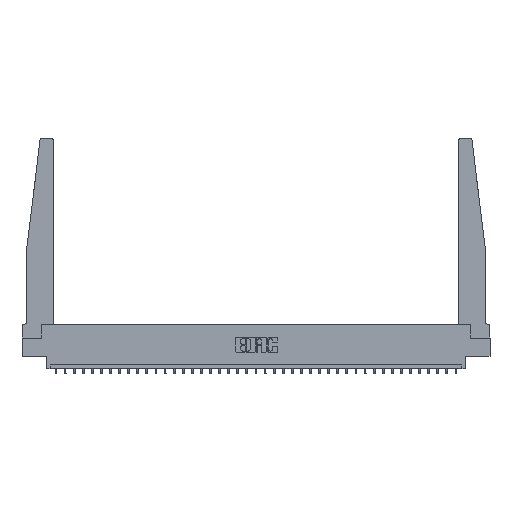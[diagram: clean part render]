
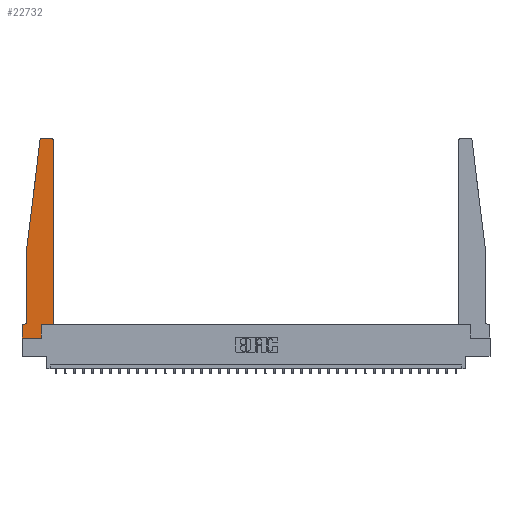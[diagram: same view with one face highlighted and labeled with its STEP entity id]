
A CAD part, top view. The second image highlights one B-rep face of the part: STEP entity #22732.
In plain terms, the highlighted planar face has unit normal (0, 0, 1).
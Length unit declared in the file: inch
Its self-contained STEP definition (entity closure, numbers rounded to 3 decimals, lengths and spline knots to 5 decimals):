
#121 = CARTESIAN_POINT ( 'NONE',  ( 0.425, 0.18, 0.37 ) ) ;
#273 = LINE ( 'NONE', #121, #26267 ) ;
#359 = ORIENTED_EDGE ( 'NONE', *, *, #1208, .T. ) ;
#466 = VERTEX_POINT ( 'NONE', #6820 ) ;
#1101 = LINE ( 'NONE', #6341, #20397 ) ;
#1208 = EDGE_CURVE ( 'NONE', #28854, #10786, #15111, .T. ) ;
#1490 = VERTEX_POINT ( 'NONE', #4313 ) ;
#1875 = CARTESIAN_POINT ( 'NONE',  ( 0.065, 0.2375, 0.37 ) ) ;
#2085 = CARTESIAN_POINT ( 'NONE',  ( 0., 0., 0.37 ) ) ;
#2220 = DIRECTION ( 'NONE',  ( 0., 1., 0. ) ) ;
#2497 = VERTEX_POINT ( 'NONE', #21222 ) ;
#3133 = CARTESIAN_POINT ( 'NONE',  ( 0., 0., 0.37 ) ) ;
#3214 = CARTESIAN_POINT ( 'NONE',  ( 0., 0., 0.37 ) ) ;
#3490 = ORIENTED_EDGE ( 'NONE', *, *, #5135, .T. ) ;
#3610 = VERTEX_POINT ( 'NONE', #25911 ) ;
#3616 = LINE ( 'NONE', #13881, #29569 ) ;
#3921 = DIRECTION ( 'NONE',  ( -1., 0., 0. ) ) ;
#4313 = CARTESIAN_POINT ( 'NONE',  ( 0.425, 0.18, 0.37 ) ) ;
#4777 = EDGE_CURVE ( 'NONE', #13607, #4840, #18002, .T. ) ;
#4840 = VERTEX_POINT ( 'NONE', #18694 ) ;
#4841 = ORIENTED_EDGE ( 'NONE', *, *, #30236, .T. ) ;
#5081 = CARTESIAN_POINT ( 'NONE',  ( 0.425, 2.72, 0.37 ) ) ;
#5135 = EDGE_CURVE ( 'NONE', #13281, #1490, #273, .T. ) ;
#5144 = ORIENTED_EDGE ( 'NONE', *, *, #21351, .T. ) ;
#5397 = CARTESIAN_POINT ( 'NONE',  ( 0.25, 2.75, 0.37 ) ) ;
#5709 = FACE_OUTER_BOUND ( 'NONE', #6802, .T. ) ;
#5917 = AXIS2_PLACEMENT_3D ( 'NONE', #26111, #11046, #28576 ) ;
#6341 = CARTESIAN_POINT ( 'NONE',  ( 0.065, 0.1875, 0.37 ) ) ;
#6802 = EDGE_LOOP ( 'NONE', ( #18828, #26869, #4841, #10801, #17477, #5144, #359, #13051, #18697, #3490, #19641, #19164 ) ) ;
#6820 = CARTESIAN_POINT ( 'NONE',  ( 0.2605, 0., 0.37 ) ) ;
#7043 = EDGE_CURVE ( 'NONE', #19220, #19482, #12801, .T. ) ;
#7483 = EDGE_CURVE ( 'NONE', #466, #13281, #32360, .T. ) ;
#7883 = VECTOR ( 'NONE', #22248, 39.37008 ) ;
#8408 = VECTOR ( 'NONE', #30812, 39.37008 ) ;
#8922 = DIRECTION ( 'NONE',  ( -0.122, -0.992, 0. ) ) ;
#9747 = CARTESIAN_POINT ( 'NONE',  ( 0.2605, 0.18, 0.37 ) ) ;
#10602 = AXIS2_PLACEMENT_3D ( 'NONE', #28550, #13560, #31067 ) ;
#10786 = VERTEX_POINT ( 'NONE', #3214 ) ;
#10801 = ORIENTED_EDGE ( 'NONE', *, *, #12232, .T. ) ;
#11046 = DIRECTION ( 'NONE',  ( 0., 0., -1. ) ) ;
#11524 = CARTESIAN_POINT ( 'NONE',  ( 0.425, 0.18, 0.37 ) ) ;
#12232 = EDGE_CURVE ( 'NONE', #3610, #13607, #22268, .T. ) ;
#12317 = VECTOR ( 'NONE', #21481, 39.37008 ) ;
#12801 = CIRCLE ( 'NONE', #15674, 0.03 ) ;
#12900 = DIRECTION ( 'NONE',  ( 0., 0., 1. ) ) ;
#13051 = ORIENTED_EDGE ( 'NONE', *, *, #31712, .T. ) ;
#13281 = VERTEX_POINT ( 'NONE', #30691 ) ;
#13484 = CARTESIAN_POINT ( 'NONE',  ( 0., 0.1875, 0.37 ) ) ;
#13560 = DIRECTION ( 'NONE',  ( 0., 0., 1. ) ) ;
#13607 = VERTEX_POINT ( 'NONE', #1875 ) ;
#13873 = EDGE_CURVE ( 'NONE', #2497, #19220, #22214, .T. ) ;
#13881 = CARTESIAN_POINT ( 'NONE',  ( 0.065, 1.25, 0.37 ) ) ;
#13954 = VECTOR ( 'NONE', #30551, 39.37008 ) ;
#13956 = CARTESIAN_POINT ( 'NONE',  ( 0.065, 1.25, 0.37 ) ) ;
#14782 = CARTESIAN_POINT ( 'NONE',  ( 0., 0.1875, 0.37 ) ) ;
#15111 = LINE ( 'NONE', #3133, #8408 ) ;
#15674 = AXIS2_PLACEMENT_3D ( 'NONE', #27889, #12900, #30377 ) ;
#16913 = LINE ( 'NONE', #2085, #7883 ) ;
#17211 = CARTESIAN_POINT ( 'NONE',  ( 0.27653, 2.75, 0.37 ) ) ;
#17277 = DIRECTION ( 'NONE',  ( 1., 0., 0. ) ) ;
#17477 = ORIENTED_EDGE ( 'NONE', *, *, #4777, .T. ) ;
#18002 = CIRCLE ( 'NONE', #5917, 0.05 ) ;
#18322 = EDGE_CURVE ( 'NONE', #25398, #2497, #27342, .T. ) ;
#18694 = CARTESIAN_POINT ( 'NONE',  ( 0.015, 0.1875, 0.37 ) ) ;
#18697 = ORIENTED_EDGE ( 'NONE', *, *, #7483, .T. ) ;
#18828 = ORIENTED_EDGE ( 'NONE', *, *, #13873, .T. ) ;
#19164 = ORIENTED_EDGE ( 'NONE', *, *, #18322, .T. ) ;
#19220 = VERTEX_POINT ( 'NONE', #17211 ) ;
#19482 = VERTEX_POINT ( 'NONE', #26022 ) ;
#19641 = ORIENTED_EDGE ( 'NONE', *, *, #25081, .T. ) ;
#19900 = AXIS2_PLACEMENT_3D ( 'NONE', #14782, #32275, #17277 ) ;
#20397 = VECTOR ( 'NONE', #3921, 39.37008 ) ;
#21222 = CARTESIAN_POINT ( 'NONE',  ( 0.395, 2.75, 0.37 ) ) ;
#21351 = EDGE_CURVE ( 'NONE', #4840, #28854, #1101, .T. ) ;
#21481 = DIRECTION ( 'NONE',  ( 0., 1., 0. ) ) ;
#22214 = LINE ( 'NONE', #5397, #13954 ) ;
#22248 = DIRECTION ( 'NONE',  ( 1., 0., 0. ) ) ;
#22268 = LINE ( 'NONE', #13956, #29695 ) ;
#22732 = ADVANCED_FACE ( 'NONE', ( #5709 ), #27272, .T. ) ;
#25081 = EDGE_CURVE ( 'NONE', #1490, #25398, #25661, .T. ) ;
#25342 = DIRECTION ( 'NONE',  ( 1., 0., 0. ) ) ;
#25398 = VERTEX_POINT ( 'NONE', #5081 ) ;
#25661 = LINE ( 'NONE', #11524, #12317 ) ;
#25772 = VECTOR ( 'NONE', #2220, 39.37008 ) ;
#25911 = CARTESIAN_POINT ( 'NONE',  ( 0.065, 1.25, 0.37 ) ) ;
#26022 = CARTESIAN_POINT ( 'NONE',  ( 0.24675, 2.72367, 0.37 ) ) ;
#26111 = CARTESIAN_POINT ( 'NONE',  ( 0.015, 0.2375, 0.37 ) ) ;
#26267 = VECTOR ( 'NONE', #25342, 39.37008 ) ;
#26869 = ORIENTED_EDGE ( 'NONE', *, *, #7043, .T. ) ;
#27272 = PLANE ( 'NONE',  #19900 ) ;
#27342 = CIRCLE ( 'NONE', #10602, 0.03 ) ;
#27889 = CARTESIAN_POINT ( 'NONE',  ( 0.27653, 2.72, 0.37 ) ) ;
#28550 = CARTESIAN_POINT ( 'NONE',  ( 0.395, 2.72, 0.37 ) ) ;
#28576 = DIRECTION ( 'NONE',  ( -1., 0., 0. ) ) ;
#28854 = VERTEX_POINT ( 'NONE', #13484 ) ;
#29569 = VECTOR ( 'NONE', #8922, 39.37008 ) ;
#29695 = VECTOR ( 'NONE', #31467, 39.37008 ) ;
#30236 = EDGE_CURVE ( 'NONE', #19482, #3610, #3616, .T. ) ;
#30377 = DIRECTION ( 'NONE',  ( 1., 0., 0. ) ) ;
#30551 = DIRECTION ( 'NONE',  ( -1., 0., 0. ) ) ;
#30691 = CARTESIAN_POINT ( 'NONE',  ( 0.2605, 0.18, 0.37 ) ) ;
#30812 = DIRECTION ( 'NONE',  ( 0., -1., 0. ) ) ;
#31067 = DIRECTION ( 'NONE',  ( 1., 0., 0. ) ) ;
#31467 = DIRECTION ( 'NONE',  ( 0., -1., 0. ) ) ;
#31712 = EDGE_CURVE ( 'NONE', #10786, #466, #16913, .T. ) ;
#32275 = DIRECTION ( 'NONE',  ( 0., 0., 1. ) ) ;
#32360 = LINE ( 'NONE', #9747, #25772 ) ;
